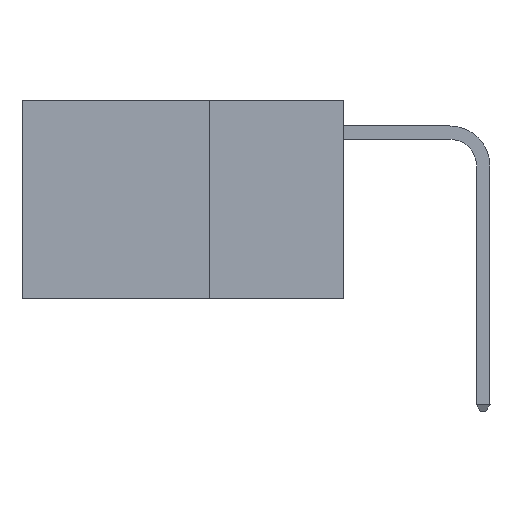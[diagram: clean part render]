
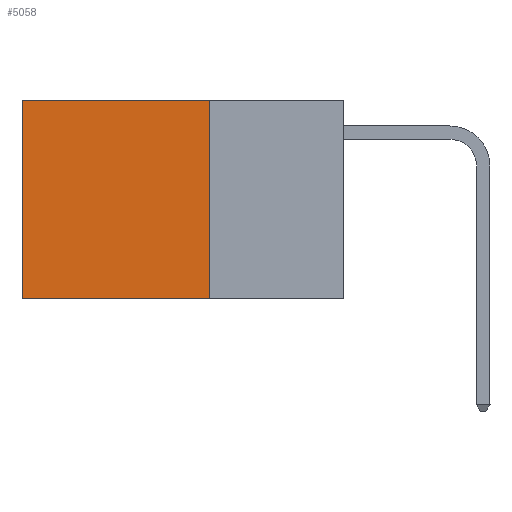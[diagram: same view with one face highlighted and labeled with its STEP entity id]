
A CAD part, left-side view. The second image highlights one B-rep face of the part: STEP entity #5058.
In plain terms, the highlighted planar face has unit normal (-1, 0, 0).
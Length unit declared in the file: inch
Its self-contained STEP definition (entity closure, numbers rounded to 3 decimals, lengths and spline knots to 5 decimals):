
#605 = ORIENTED_EDGE ( 'NONE', *, *, #13420, .F. ) ;
#773 = EDGE_LOOP ( 'NONE', ( #10343, #9050, #605, #11666 ) ) ;
#1093 = VERTEX_POINT ( 'NONE', #10036 ) ;
#1828 = VECTOR ( 'NONE', #1976, 39.37008 ) ;
#1976 = DIRECTION ( 'NONE',  ( 0., 0., -1. ) ) ;
#2028 = CARTESIAN_POINT ( 'NONE',  ( 0.2625, 0.25, 0. ) ) ;
#2326 = CARTESIAN_POINT ( 'NONE',  ( 0.2625, 0.6, 0. ) ) ;
#3055 = VERTEX_POINT ( 'NONE', #3135 ) ;
#3135 = CARTESIAN_POINT ( 'NONE',  ( 0.2625, 0.6, 0. ) ) ;
#3158 = VECTOR ( 'NONE', #3430, 39.37008 ) ;
#3430 = DIRECTION ( 'NONE',  ( 0., 1., 0. ) ) ;
#3649 = EDGE_CURVE ( 'NONE', #3055, #4332, #7974, .T. ) ;
#4332 = VERTEX_POINT ( 'NONE', #8455 ) ;
#4405 = VECTOR ( 'NONE', #6480, 39.37008 ) ;
#4967 = EDGE_CURVE ( 'NONE', #1093, #4332, #14373, .T. ) ;
#5058 = ADVANCED_FACE ( 'NONE', ( #13348 ), #5418, .F. ) ;
#5188 = LINE ( 'NONE', #5332, #1828 ) ;
#5332 = CARTESIAN_POINT ( 'NONE',  ( 0.2625, 0.25, 0. ) ) ;
#5418 = PLANE ( 'NONE',  #6678 ) ;
#5892 = CARTESIAN_POINT ( 'NONE',  ( 0.2625, 0.25, 0. ) ) ;
#6480 = DIRECTION ( 'NONE',  ( 0., 1., 0. ) ) ;
#6678 = AXIS2_PLACEMENT_3D ( 'NONE', #9912, #14310, #8792 ) ;
#6737 = CARTESIAN_POINT ( 'NONE',  ( 0.2625, 0.25, -0.37 ) ) ;
#7974 = LINE ( 'NONE', #2326, #13882 ) ;
#8455 = CARTESIAN_POINT ( 'NONE',  ( 0.2625, 0.6, -0.37 ) ) ;
#8680 = LINE ( 'NONE', #2028, #4405 ) ;
#8792 = DIRECTION ( 'NONE',  ( 0., 0., -1. ) ) ;
#8828 = VERTEX_POINT ( 'NONE', #5892 ) ;
#9050 = ORIENTED_EDGE ( 'NONE', *, *, #4967, .F. ) ;
#9912 = CARTESIAN_POINT ( 'NONE',  ( 0.2625, 0.25, 0. ) ) ;
#10036 = CARTESIAN_POINT ( 'NONE',  ( 0.2625, 0.25, -0.37 ) ) ;
#10337 = DIRECTION ( 'NONE',  ( 0., 0., -1. ) ) ;
#10343 = ORIENTED_EDGE ( 'NONE', *, *, #3649, .T. ) ;
#11666 = ORIENTED_EDGE ( 'NONE', *, *, #13865, .T. ) ;
#13348 = FACE_OUTER_BOUND ( 'NONE', #773, .T. ) ;
#13420 = EDGE_CURVE ( 'NONE', #8828, #1093, #5188, .T. ) ;
#13865 = EDGE_CURVE ( 'NONE', #8828, #3055, #8680, .T. ) ;
#13882 = VECTOR ( 'NONE', #10337, 39.37008 ) ;
#14310 = DIRECTION ( 'NONE',  ( 1., 0., 0. ) ) ;
#14373 = LINE ( 'NONE', #6737, #3158 ) ;
